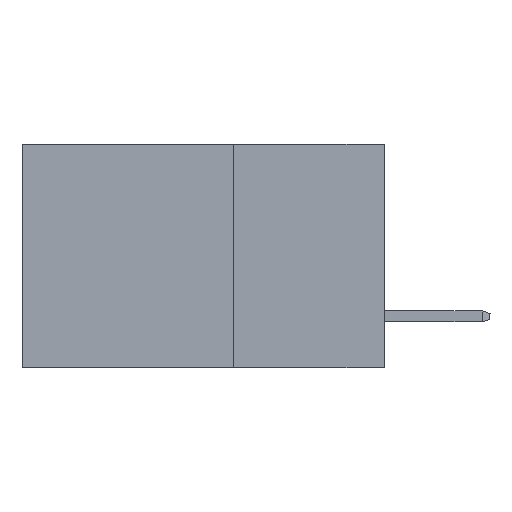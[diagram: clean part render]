
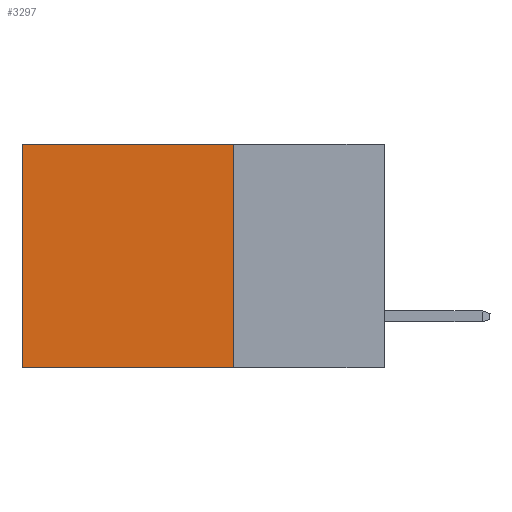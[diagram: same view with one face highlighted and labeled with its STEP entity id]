
A CAD part, left-side view. The second image highlights one B-rep face of the part: STEP entity #3297.
In plain terms, the highlighted planar face has unit normal (-1, 0, 0).
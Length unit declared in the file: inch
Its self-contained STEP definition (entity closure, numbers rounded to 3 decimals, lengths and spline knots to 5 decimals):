
#290 = AXIS2_PLACEMENT_3D ( 'NONE', #6877, #11034, #544 ) ;
#544 = DIRECTION ( 'NONE',  ( 0., 0., -1. ) ) ;
#1090 = EDGE_CURVE ( 'NONE', #2590, #2004, #4863, .T. ) ;
#2004 = VERTEX_POINT ( 'NONE', #9716 ) ;
#2236 = FACE_OUTER_BOUND ( 'NONE', #8605, .T. ) ;
#2266 = CARTESIAN_POINT ( 'NONE',  ( 0.2615, 0.25, -0.37 ) ) ;
#2575 = CARTESIAN_POINT ( 'NONE',  ( 0.2615, 0.25, -0.37 ) ) ;
#2590 = VERTEX_POINT ( 'NONE', #6780 ) ;
#3297 = ADVANCED_FACE ( 'NONE', ( #2236 ), #6400, .F. ) ;
#3343 = EDGE_CURVE ( 'NONE', #13360, #2004, #6813, .T. ) ;
#3402 = EDGE_CURVE ( 'NONE', #6235, #13360, #11927, .T. ) ;
#3434 = VECTOR ( 'NONE', #10960, 39.37008 ) ;
#4863 = LINE ( 'NONE', #8752, #9066 ) ;
#5206 = ORIENTED_EDGE ( 'NONE', *, *, #3343, .F. ) ;
#5440 = VECTOR ( 'NONE', #9264, 39.37008 ) ;
#5723 = DIRECTION ( 'NONE',  ( 0., 0., -1. ) ) ;
#5985 = CARTESIAN_POINT ( 'NONE',  ( 0.2615, 0.25, 0. ) ) ;
#6058 = ORIENTED_EDGE ( 'NONE', *, *, #3402, .F. ) ;
#6235 = VERTEX_POINT ( 'NONE', #10078 ) ;
#6400 = PLANE ( 'NONE',  #290 ) ;
#6780 = CARTESIAN_POINT ( 'NONE',  ( 0.2615, 0.6, 0. ) ) ;
#6813 = LINE ( 'NONE', #12054, #3434 ) ;
#6877 = CARTESIAN_POINT ( 'NONE',  ( 0.2615, 0.25, -0.37 ) ) ;
#8605 = EDGE_LOOP ( 'NONE', ( #10661, #5206, #6058, #12968 ) ) ;
#8752 = CARTESIAN_POINT ( 'NONE',  ( 0.2615, 0.6, -0.37 ) ) ;
#9066 = VECTOR ( 'NONE', #9834, 39.37008 ) ;
#9264 = DIRECTION ( 'NONE',  ( 0., 1., 0. ) ) ;
#9634 = EDGE_CURVE ( 'NONE', #6235, #2590, #10023, .T. ) ;
#9716 = CARTESIAN_POINT ( 'NONE',  ( 0.2615, 0.6, -0.37 ) ) ;
#9834 = DIRECTION ( 'NONE',  ( 0., 0., -1. ) ) ;
#10023 = LINE ( 'NONE', #5985, #5440 ) ;
#10078 = CARTESIAN_POINT ( 'NONE',  ( 0.2615, 0.25, 0. ) ) ;
#10637 = VECTOR ( 'NONE', #5723, 39.37008 ) ;
#10661 = ORIENTED_EDGE ( 'NONE', *, *, #1090, .T. ) ;
#10960 = DIRECTION ( 'NONE',  ( 0., 1., 0. ) ) ;
#11034 = DIRECTION ( 'NONE',  ( 1., 0., 0. ) ) ;
#11927 = LINE ( 'NONE', #2575, #10637 ) ;
#12054 = CARTESIAN_POINT ( 'NONE',  ( 0.2615, 0.25, -0.37 ) ) ;
#12968 = ORIENTED_EDGE ( 'NONE', *, *, #9634, .T. ) ;
#13360 = VERTEX_POINT ( 'NONE', #2266 ) ;
